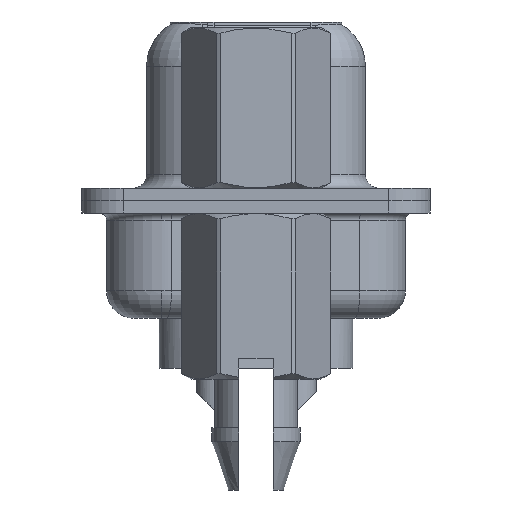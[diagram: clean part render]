
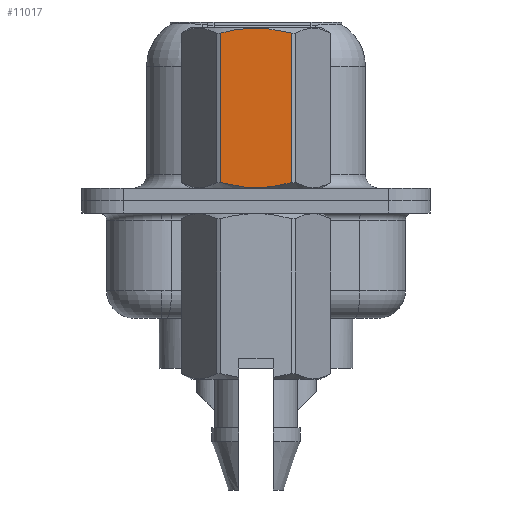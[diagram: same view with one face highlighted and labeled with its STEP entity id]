
A CAD part, left-side view. The second image highlights one B-rep face of the part: STEP entity #11017.
In plain terms, the highlighted planar face has unit normal (-1, 0, 0).
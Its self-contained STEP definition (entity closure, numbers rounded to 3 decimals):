
#344 = CARTESIAN_POINT ( 'NONE',  ( -2.381, 0.215, 0.468 ) ) ;
#399 = B_SPLINE_CURVE_WITH_KNOTS ( 'NONE', 3,
 ( #10616, #12910, #5041, #16494, #13032, #4916, #3145, #8716, #18754, #20773 ),
 .UNSPECIFIED., .F., .F.,
 ( 4, 2, 2, 2, 4 ),
 ( 0.001, 0.002, 0.002, 0.003, 0.004 ),
 .UNSPECIFIED. ) ;
#448 = VECTOR ( 'NONE', #19365, 1000. ) ;
#1393 = ORIENTED_EDGE ( 'NONE', *, *, #5190, .T. ) ;
#2040 = DIRECTION ( 'NONE',  ( -1., 0., 0. ) ) ;
#2102 = CARTESIAN_POINT ( 'NONE',  ( -2.381, -0.432, 0.485 ) ) ;
#2377 = B_SPLINE_CURVE_WITH_KNOTS ( 'NONE', 3,
 ( #23322, #15946, #14047, #19506, #344, #13794, #2102, #13670, #21796, #21410 ),
 .UNSPECIFIED., .F., .F.,
 ( 4, 2, 2, 2, 4 ),
 ( 0.003, 0.003, 0.004, 0.004, 0.005 ),
 .UNSPECIFIED. ) ;
#3005 = ORIENTED_EDGE ( 'NONE', *, *, #8795, .T. ) ;
#3145 = CARTESIAN_POINT ( 'NONE',  ( -2.381, 0.428, 6.215 ) ) ;
#4916 = CARTESIAN_POINT ( 'NONE',  ( -2.381, 0.215, 6.232 ) ) ;
#5041 = CARTESIAN_POINT ( 'NONE',  ( -2.381, -0.858, 6.15 ) ) ;
#5114 = EDGE_LOOP ( 'NONE', ( #3005, #14203, #1393, #14766 ) ) ;
#5190 = EDGE_CURVE ( 'NONE', #22957, #7279, #399, .T. ) ;
#6786 = CARTESIAN_POINT ( 'NONE',  ( -2.381, 1.273, 6.048 ) ) ;
#7279 = VERTEX_POINT ( 'NONE', #6786 ) ;
#8716 = CARTESIAN_POINT ( 'NONE',  ( -2.381, 0.853, 6.151 ) ) ;
#8795 = EDGE_CURVE ( 'NONE', #22790, #11709, #2377, .T. ) ;
#9030 = LINE ( 'NONE', #16820, #15110 ) ;
#9685 = CARTESIAN_POINT ( 'NONE',  ( -2.381, -1.273, 3.792 ) ) ;
#9755 = DIRECTION ( 'NONE',  ( 0., -1., 0. ) ) ;
#10616 = CARTESIAN_POINT ( 'NONE',  ( -2.381, -1.273, 6.048 ) ) ;
#11017 = ADVANCED_FACE ( 'NONE', ( #11688 ), #19441, .T. ) ;
#11688 = FACE_OUTER_BOUND ( 'NONE', #5114, .T. ) ;
#11709 = VERTEX_POINT ( 'NONE', #22135 ) ;
#12910 = CARTESIAN_POINT ( 'NONE',  ( -2.381, -1.066, 6.104 ) ) ;
#12988 = DIRECTION ( 'NONE',  ( 0., 0., -1. ) ) ;
#13032 = CARTESIAN_POINT ( 'NONE',  ( -2.381, -0.215, 6.232 ) ) ;
#13515 = LINE ( 'NONE', #9685, #448 ) ;
#13670 = CARTESIAN_POINT ( 'NONE',  ( -2.381, -0.858, 0.55 ) ) ;
#13764 = CARTESIAN_POINT ( 'NONE',  ( -2.381, 1.273, 0.652 ) ) ;
#13794 = CARTESIAN_POINT ( 'NONE',  ( -2.381, -0.215, 0.468 ) ) ;
#14047 = CARTESIAN_POINT ( 'NONE',  ( -2.381, 0.853, 0.549 ) ) ;
#14203 = ORIENTED_EDGE ( 'NONE', *, *, #21685, .T. ) ;
#14766 = ORIENTED_EDGE ( 'NONE', *, *, #22733, .T. ) ;
#15110 = VECTOR ( 'NONE', #12988, 1000. ) ;
#15946 = CARTESIAN_POINT ( 'NONE',  ( -2.381, 1.065, 0.596 ) ) ;
#16494 = CARTESIAN_POINT ( 'NONE',  ( -2.381, -0.432, 6.215 ) ) ;
#16820 = CARTESIAN_POINT ( 'NONE',  ( -2.381, 1.273, 3.792 ) ) ;
#17030 = CARTESIAN_POINT ( 'NONE',  ( -2.381, 1.375, -3.75 ) ) ;
#18754 = CARTESIAN_POINT ( 'NONE',  ( -2.381, 1.065, 6.104 ) ) ;
#19365 = DIRECTION ( 'NONE',  ( 0., 0., 1. ) ) ;
#19441 = PLANE ( 'NONE',  #21682 ) ;
#19506 = CARTESIAN_POINT ( 'NONE',  ( -2.381, 0.428, 0.485 ) ) ;
#20773 = CARTESIAN_POINT ( 'NONE',  ( -2.381, 1.273, 6.048 ) ) ;
#21410 = CARTESIAN_POINT ( 'NONE',  ( -2.381, -1.273, 0.652 ) ) ;
#21682 = AXIS2_PLACEMENT_3D ( 'NONE', #17030, #2040, #9755 ) ;
#21685 = EDGE_CURVE ( 'NONE', #11709, #22957, #13515, .T. ) ;
#21796 = CARTESIAN_POINT ( 'NONE',  ( -2.381, -1.066, 0.596 ) ) ;
#22135 = CARTESIAN_POINT ( 'NONE',  ( -2.381, -1.273, 0.652 ) ) ;
#22733 = EDGE_CURVE ( 'NONE', #7279, #22790, #9030, .T. ) ;
#22790 = VERTEX_POINT ( 'NONE', #13764 ) ;
#22957 = VERTEX_POINT ( 'NONE', #23285 ) ;
#23285 = CARTESIAN_POINT ( 'NONE',  ( -2.381, -1.273, 6.048 ) ) ;
#23322 = CARTESIAN_POINT ( 'NONE',  ( -2.381, 1.273, 0.652 ) ) ;
